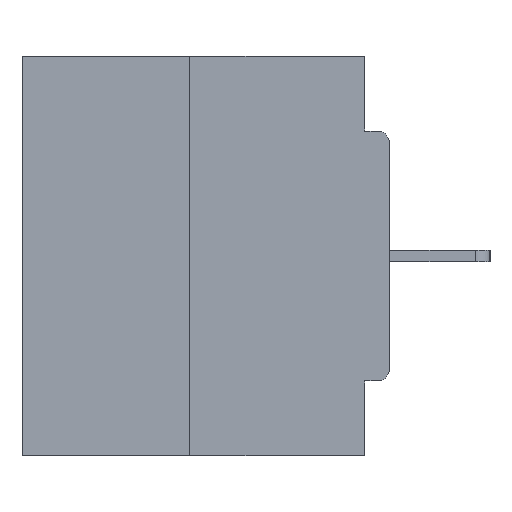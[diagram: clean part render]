
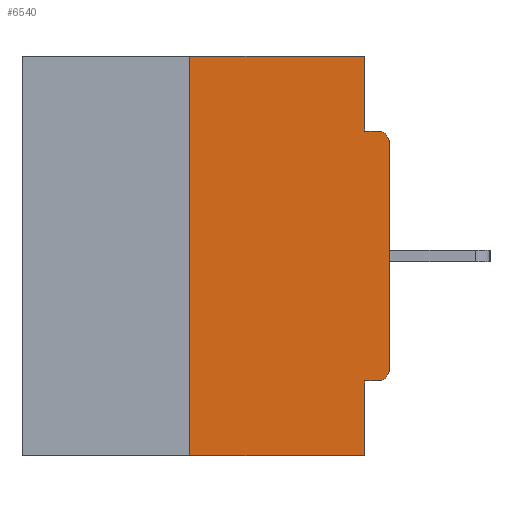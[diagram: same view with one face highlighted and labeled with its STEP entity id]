
A CAD part, left-side view. The second image highlights one B-rep face of the part: STEP entity #6540.
In plain terms, the highlighted planar face has unit normal (-1, 0, 0).
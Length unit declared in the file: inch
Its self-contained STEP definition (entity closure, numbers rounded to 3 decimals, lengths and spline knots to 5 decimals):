
#284 = CARTESIAN_POINT ( 'NONE',  ( 0., 0.25, 0. ) ) ;
#482 = DIRECTION ( 'NONE',  ( 1., 0., 0. ) ) ;
#635 = CARTESIAN_POINT ( 'NONE',  ( 0., 0.015, -0.0935 ) ) ;
#639 = CARTESIAN_POINT ( 'NONE',  ( 0., 0.46, -0.5 ) ) ;
#688 = VERTEX_POINT ( 'NONE', #16923 ) ;
#1023 = CARTESIAN_POINT ( 'NONE',  ( 0., 0., 0. ) ) ;
#1670 = DIRECTION ( 'NONE',  ( 0., 0., 1. ) ) ;
#2503 = CARTESIAN_POINT ( 'NONE',  ( 0., 0.46, 0. ) ) ;
#3200 = CARTESIAN_POINT ( 'NONE',  ( 0., 0.031, -0.4065 ) ) ;
#3300 = EDGE_CURVE ( 'NONE', #24536, #14776, #10087, .T. ) ;
#3393 = ORIENTED_EDGE ( 'NONE', *, *, #3300, .F. ) ;
#4020 = DIRECTION ( 'NONE',  ( -1., 0., 0. ) ) ;
#4108 = AXIS2_PLACEMENT_3D ( 'NONE', #26818, #482, #15952 ) ;
#4719 = AXIS2_PLACEMENT_3D ( 'NONE', #9859, #12162, #16171 ) ;
#4944 = ORIENTED_EDGE ( 'NONE', *, *, #19515, .T. ) ;
#5652 = CARTESIAN_POINT ( 'NONE',  ( 0., 0., -0.0935 ) ) ;
#5925 = DIRECTION ( 'NONE',  ( 0., 1., 0. ) ) ;
#6540 = ADVANCED_FACE ( 'NONE', ( #7209 ), #6652, .F. ) ;
#6652 = PLANE ( 'NONE',  #4108 ) ;
#7209 = FACE_OUTER_BOUND ( 'NONE', #8422, .T. ) ;
#7401 = CARTESIAN_POINT ( 'NONE',  ( 0., 0.031, -0.5 ) ) ;
#7492 = VECTOR ( 'NONE', #1670, 39.37008 ) ;
#7895 = LINE ( 'NONE', #18773, #14929 ) ;
#8077 = DIRECTION ( 'NONE',  ( 0., -1., 0. ) ) ;
#8422 = EDGE_LOOP ( 'NONE', ( #8688, #21831, #18468, #12193, #22845, #12795, #4944, #19220, #3393, #17852 ) ) ;
#8688 = ORIENTED_EDGE ( 'NONE', *, *, #19023, .F. ) ;
#9282 = EDGE_CURVE ( 'NONE', #19897, #11980, #16802, .T. ) ;
#9859 = CARTESIAN_POINT ( 'NONE',  ( 0., 0.015, -0.1085 ) ) ;
#9864 = CARTESIAN_POINT ( 'NONE',  ( 0., 0., -0.3915 ) ) ;
#9971 = DIRECTION ( 'NONE',  ( 0., 0., -1. ) ) ;
#10087 = LINE ( 'NONE', #5652, #13192 ) ;
#10115 = EDGE_CURVE ( 'NONE', #24909, #12559, #21389, .T. ) ;
#10146 = VECTOR ( 'NONE', #9971, 39.37008 ) ;
#10177 = VECTOR ( 'NONE', #5925, 39.37008 ) ;
#10520 = CARTESIAN_POINT ( 'NONE',  ( 0., 0., -0.1085 ) ) ;
#10540 = CARTESIAN_POINT ( 'NONE',  ( 0., 0.25, 0. ) ) ;
#11045 = CARTESIAN_POINT ( 'NONE',  ( 0., 0.031, -0.0935 ) ) ;
#11980 = VERTEX_POINT ( 'NONE', #3200 ) ;
#12162 = DIRECTION ( 'NONE',  ( -1., 0., 0. ) ) ;
#12193 = ORIENTED_EDGE ( 'NONE', *, *, #15704, .F. ) ;
#12434 = CARTESIAN_POINT ( 'NONE',  ( 0., 0.031, 0. ) ) ;
#12559 = VERTEX_POINT ( 'NONE', #284 ) ;
#12795 = ORIENTED_EDGE ( 'NONE', *, *, #23399, .T. ) ;
#12861 = VERTEX_POINT ( 'NONE', #9864 ) ;
#13192 = VECTOR ( 'NONE', #8077, 39.37008 ) ;
#13417 = CIRCLE ( 'NONE', #4719, 0.015 ) ;
#13714 = CARTESIAN_POINT ( 'NONE',  ( 0., 0.015, -0.4065 ) ) ;
#14104 = VERTEX_POINT ( 'NONE', #12434 ) ;
#14776 = VERTEX_POINT ( 'NONE', #635 ) ;
#14841 = VECTOR ( 'NONE', #22472, 39.37008 ) ;
#14929 = VECTOR ( 'NONE', #16921, 39.37008 ) ;
#15410 = DIRECTION ( 'NONE',  ( 0., -1., 0. ) ) ;
#15482 = CARTESIAN_POINT ( 'NONE',  ( 0., 0.015, -0.3915 ) ) ;
#15704 = EDGE_CURVE ( 'NONE', #11980, #688, #18418, .T. ) ;
#15952 = DIRECTION ( 'NONE',  ( 0., 0., -1. ) ) ;
#16171 = DIRECTION ( 'NONE',  ( 0., 0., -1. ) ) ;
#16748 = CIRCLE ( 'NONE', #24046, 0.015 ) ;
#16802 = LINE ( 'NONE', #25522, #10177 ) ;
#16921 = DIRECTION ( 'NONE',  ( 0., 0., -1. ) ) ;
#16923 = CARTESIAN_POINT ( 'NONE',  ( 0., 0.031, -0.5 ) ) ;
#17195 = DIRECTION ( 'NONE',  ( 0., 0., -1. ) ) ;
#17852 = ORIENTED_EDGE ( 'NONE', *, *, #23149, .F. ) ;
#17995 = VECTOR ( 'NONE', #24104, 39.37008 ) ;
#18418 = LINE ( 'NONE', #7401, #10146 ) ;
#18465 = EDGE_CURVE ( 'NONE', #26923, #14776, #13417, .T. ) ;
#18468 = ORIENTED_EDGE ( 'NONE', *, *, #20258, .T. ) ;
#18773 = CARTESIAN_POINT ( 'NONE',  ( 0., 0.031, 0. ) ) ;
#19023 = EDGE_CURVE ( 'NONE', #12559, #14104, #24388, .T. ) ;
#19220 = ORIENTED_EDGE ( 'NONE', *, *, #18465, .T. ) ;
#19515 = EDGE_CURVE ( 'NONE', #12861, #26923, #27352, .T. ) ;
#19897 = VERTEX_POINT ( 'NONE', #13714 ) ;
#20258 = EDGE_CURVE ( 'NONE', #24909, #688, #24532, .T. ) ;
#21284 = CARTESIAN_POINT ( 'NONE',  ( 0., 0.25, -0.5 ) ) ;
#21389 = LINE ( 'NONE', #10540, #7492 ) ;
#21831 = ORIENTED_EDGE ( 'NONE', *, *, #10115, .F. ) ;
#22472 = DIRECTION ( 'NONE',  ( 0., 0., 1. ) ) ;
#22845 = ORIENTED_EDGE ( 'NONE', *, *, #9282, .F. ) ;
#23058 = VECTOR ( 'NONE', #15410, 39.37008 ) ;
#23149 = EDGE_CURVE ( 'NONE', #14104, #24536, #7895, .T. ) ;
#23399 = EDGE_CURVE ( 'NONE', #19897, #12861, #16748, .T. ) ;
#24046 = AXIS2_PLACEMENT_3D ( 'NONE', #15482, #4020, #17195 ) ;
#24104 = DIRECTION ( 'NONE',  ( 0., -1., 0. ) ) ;
#24388 = LINE ( 'NONE', #2503, #17995 ) ;
#24532 = LINE ( 'NONE', #639, #23058 ) ;
#24536 = VERTEX_POINT ( 'NONE', #11045 ) ;
#24909 = VERTEX_POINT ( 'NONE', #21284 ) ;
#25522 = CARTESIAN_POINT ( 'NONE',  ( 0., 0., -0.4065 ) ) ;
#26818 = CARTESIAN_POINT ( 'NONE',  ( 0., 0.46, 0. ) ) ;
#26923 = VERTEX_POINT ( 'NONE', #10520 ) ;
#27352 = LINE ( 'NONE', #1023, #14841 ) ;
